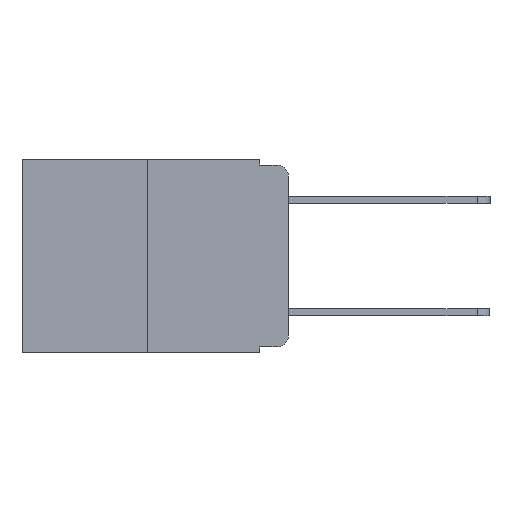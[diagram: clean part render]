
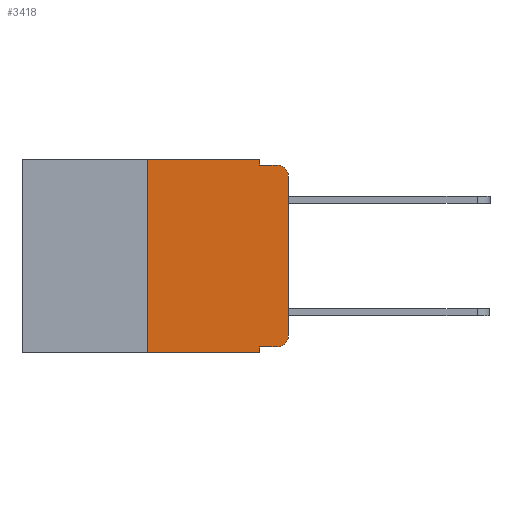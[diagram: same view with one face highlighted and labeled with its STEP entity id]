
A CAD part, left-side view. The second image highlights one B-rep face of the part: STEP entity #3418.
In plain terms, the highlighted planar face has unit normal (-1, 0, 0).
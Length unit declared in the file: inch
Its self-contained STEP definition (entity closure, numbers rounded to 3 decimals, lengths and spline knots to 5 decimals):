
#560 = ORIENTED_EDGE ( 'NONE', *, *, #3220, .T. ) ;
#1123 = LINE ( 'NONE', #1841, #7554 ) ;
#1187 = CARTESIAN_POINT ( 'NONE',  ( 0., 0.051, -0.343 ) ) ;
#1432 = VECTOR ( 'NONE', #9546, 39.37008 ) ;
#1526 = CIRCLE ( 'NONE', #7396, 0.02 ) ;
#1574 = EDGE_CURVE ( 'NONE', #14298, #9285, #1123, .T. ) ;
#1841 = CARTESIAN_POINT ( 'NONE',  ( 0., 0.473, -0.343 ) ) ;
#2371 = ORIENTED_EDGE ( 'NONE', *, *, #10488, .T. ) ;
#2521 = CARTESIAN_POINT ( 'NONE',  ( 0., 0.051, -0.01 ) ) ;
#2568 = DIRECTION ( 'NONE',  ( 0., -1., 0. ) ) ;
#2743 = CARTESIAN_POINT ( 'NONE',  ( 0., 0.02, -0.333 ) ) ;
#3119 = CIRCLE ( 'NONE', #8248, 0.02 ) ;
#3176 = CARTESIAN_POINT ( 'NONE',  ( 0., 0.051, 0. ) ) ;
#3220 = EDGE_CURVE ( 'NONE', #15723, #3945, #3119, .T. ) ;
#3271 = CARTESIAN_POINT ( 'NONE',  ( 0., 0.051, -0.333 ) ) ;
#3418 = ADVANCED_FACE ( 'NONE', ( #12772 ), #13256, .F. ) ;
#3495 = DIRECTION ( 'NONE',  ( 1., 0., 0. ) ) ;
#3514 = LINE ( 'NONE', #12497, #12583 ) ;
#3647 = EDGE_CURVE ( 'NONE', #10909, #13310, #3514, .T. ) ;
#3653 = DIRECTION ( 'NONE',  ( 0., 0., 1. ) ) ;
#3695 = AXIS2_PLACEMENT_3D ( 'NONE', #10973, #3495, #12143 ) ;
#3738 = VERTEX_POINT ( 'NONE', #2743 ) ;
#3826 = ORIENTED_EDGE ( 'NONE', *, *, #3647, .F. ) ;
#3945 = VERTEX_POINT ( 'NONE', #4432 ) ;
#3985 = VECTOR ( 'NONE', #4413, 39.37008 ) ;
#4413 = DIRECTION ( 'NONE',  ( 0., 0., -1. ) ) ;
#4432 = CARTESIAN_POINT ( 'NONE',  ( 0., 0.02, -0.01 ) ) ;
#4788 = DIRECTION ( 'NONE',  ( -1., 0., 0. ) ) ;
#4961 = EDGE_CURVE ( 'NONE', #9644, #3738, #8244, .T. ) ;
#5471 = CARTESIAN_POINT ( 'NONE',  ( 0., 0.25, 0. ) ) ;
#6242 = VECTOR ( 'NONE', #14176, 39.37008 ) ;
#6441 = ORIENTED_EDGE ( 'NONE', *, *, #12636, .F. ) ;
#6593 = DIRECTION ( 'NONE',  ( 0., 0., -1. ) ) ;
#6738 = CARTESIAN_POINT ( 'NONE',  ( 0., 0.051, 0. ) ) ;
#6810 = DIRECTION ( 'NONE',  ( 0., -1., 0. ) ) ;
#7117 = VECTOR ( 'NONE', #15357, 39.37008 ) ;
#7140 = CARTESIAN_POINT ( 'NONE',  ( 0., 0.25, 0. ) ) ;
#7273 = DIRECTION ( 'NONE',  ( -1., 0., 0. ) ) ;
#7396 = AXIS2_PLACEMENT_3D ( 'NONE', #14384, #7273, #15501 ) ;
#7453 = CARTESIAN_POINT ( 'NONE',  ( 0., 0., 0. ) ) ;
#7505 = EDGE_CURVE ( 'NONE', #3738, #8195, #1526, .T. ) ;
#7554 = VECTOR ( 'NONE', #6810, 39.37008 ) ;
#7604 = ORIENTED_EDGE ( 'NONE', *, *, #10284, .F. ) ;
#7689 = LINE ( 'NONE', #7453, #10561 ) ;
#7822 = EDGE_CURVE ( 'NONE', #9644, #9285, #13732, .T. ) ;
#8195 = VERTEX_POINT ( 'NONE', #11387 ) ;
#8244 = LINE ( 'NONE', #3271, #1432 ) ;
#8248 = AXIS2_PLACEMENT_3D ( 'NONE', #12142, #4788, #13316 ) ;
#9088 = CARTESIAN_POINT ( 'NONE',  ( 0., 0.051, 0. ) ) ;
#9285 = VERTEX_POINT ( 'NONE', #1187 ) ;
#9414 = EDGE_LOOP ( 'NONE', ( #2371, #560, #15141, #6441, #3826, #7604, #14625, #14966, #13039, #14108 ) ) ;
#9546 = DIRECTION ( 'NONE',  ( 0., -1., 0. ) ) ;
#9644 = VERTEX_POINT ( 'NONE', #13069 ) ;
#10284 = EDGE_CURVE ( 'NONE', #14298, #10909, #10391, .T. ) ;
#10391 = LINE ( 'NONE', #7140, #7117 ) ;
#10488 = EDGE_CURVE ( 'NONE', #8195, #15723, #7689, .T. ) ;
#10561 = VECTOR ( 'NONE', #3653, 39.37008 ) ;
#10794 = CARTESIAN_POINT ( 'NONE',  ( 0., 0., -0.03 ) ) ;
#10909 = VERTEX_POINT ( 'NONE', #5471 ) ;
#10940 = VECTOR ( 'NONE', #6593, 39.37008 ) ;
#10973 = CARTESIAN_POINT ( 'NONE',  ( 0., 0.473, 0. ) ) ;
#11312 = LINE ( 'NONE', #9088, #10940 ) ;
#11387 = CARTESIAN_POINT ( 'NONE',  ( 0., 0., -0.313 ) ) ;
#12142 = CARTESIAN_POINT ( 'NONE',  ( 0., 0.02, -0.03 ) ) ;
#12143 = DIRECTION ( 'NONE',  ( 0., 0., -1. ) ) ;
#12497 = CARTESIAN_POINT ( 'NONE',  ( 0., 0.473, 0. ) ) ;
#12529 = VERTEX_POINT ( 'NONE', #2521 ) ;
#12583 = VECTOR ( 'NONE', #2568, 39.37008 ) ;
#12636 = EDGE_CURVE ( 'NONE', #13310, #12529, #11312, .T. ) ;
#12690 = LINE ( 'NONE', #13036, #6242 ) ;
#12772 = FACE_OUTER_BOUND ( 'NONE', #9414, .T. ) ;
#13036 = CARTESIAN_POINT ( 'NONE',  ( 0., 0.051, -0.01 ) ) ;
#13039 = ORIENTED_EDGE ( 'NONE', *, *, #4961, .T. ) ;
#13069 = CARTESIAN_POINT ( 'NONE',  ( 0., 0.051, -0.333 ) ) ;
#13256 = PLANE ( 'NONE',  #3695 ) ;
#13310 = VERTEX_POINT ( 'NONE', #6738 ) ;
#13316 = DIRECTION ( 'NONE',  ( 0., 0., -1. ) ) ;
#13693 = CARTESIAN_POINT ( 'NONE',  ( 0., 0.25, -0.343 ) ) ;
#13732 = LINE ( 'NONE', #3176, #3985 ) ;
#14108 = ORIENTED_EDGE ( 'NONE', *, *, #7505, .T. ) ;
#14176 = DIRECTION ( 'NONE',  ( 0., -1., 0. ) ) ;
#14298 = VERTEX_POINT ( 'NONE', #13693 ) ;
#14384 = CARTESIAN_POINT ( 'NONE',  ( 0., 0.02, -0.313 ) ) ;
#14625 = ORIENTED_EDGE ( 'NONE', *, *, #1574, .T. ) ;
#14966 = ORIENTED_EDGE ( 'NONE', *, *, #7822, .F. ) ;
#15141 = ORIENTED_EDGE ( 'NONE', *, *, #15667, .F. ) ;
#15357 = DIRECTION ( 'NONE',  ( 0., 0., 1. ) ) ;
#15501 = DIRECTION ( 'NONE',  ( 0., 0., -1. ) ) ;
#15667 = EDGE_CURVE ( 'NONE', #12529, #3945, #12690, .T. ) ;
#15723 = VERTEX_POINT ( 'NONE', #10794 ) ;
